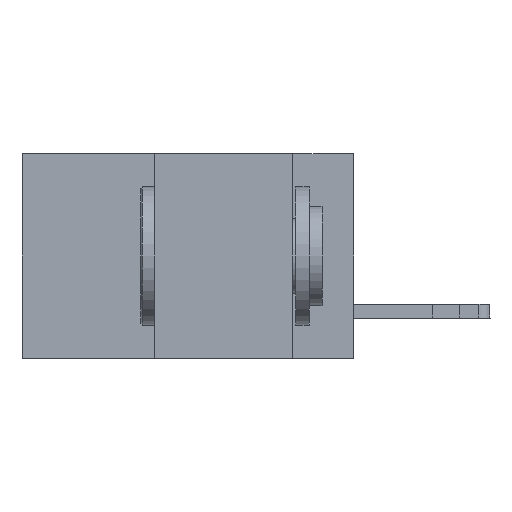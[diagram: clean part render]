
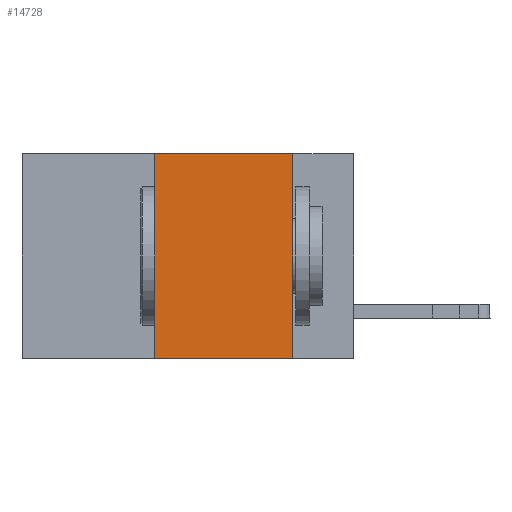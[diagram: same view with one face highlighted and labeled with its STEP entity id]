
A CAD part, left-side view. The second image highlights one B-rep face of the part: STEP entity #14728.
In plain terms, the highlighted planar face has unit normal (-1, 0, 0).
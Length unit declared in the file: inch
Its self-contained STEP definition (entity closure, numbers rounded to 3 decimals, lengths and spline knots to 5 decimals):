
#1623 = DIRECTION ( 'NONE',  ( 1., 0., 0. ) ) ;
#1757 = AXIS2_PLACEMENT_3D ( 'NONE', #15663, #1623, #9814 ) ;
#1800 = VECTOR ( 'NONE', #20126, 39.37008 ) ;
#3189 = LINE ( 'NONE', #13728, #12115 ) ;
#3239 = ORIENTED_EDGE ( 'NONE', *, *, #13617, .F. ) ;
#3322 = LINE ( 'NONE', #13503, #13799 ) ;
#3452 = EDGE_CURVE ( 'NONE', #20125, #24750, #3322, .T. ) ;
#4937 = EDGE_LOOP ( 'NONE', ( #3239, #13744, #5851, #11400 ) ) ;
#5851 = ORIENTED_EDGE ( 'NONE', *, *, #20965, .F. ) ;
#6671 = LINE ( 'NONE', #15623, #1800 ) ;
#7636 = DIRECTION ( 'NONE',  ( 0., -1., 0. ) ) ;
#9814 = DIRECTION ( 'NONE',  ( 0., 0., -1. ) ) ;
#10071 = FACE_OUTER_BOUND ( 'NONE', #4937, .T. ) ;
#11400 = ORIENTED_EDGE ( 'NONE', *, *, #3452, .T. ) ;
#12115 = VECTOR ( 'NONE', #15627, 39.37008 ) ;
#13503 = CARTESIAN_POINT ( 'NONE',  ( 0., 0.6, -0.37 ) ) ;
#13617 = EDGE_CURVE ( 'NONE', #23553, #24750, #6671, .T. ) ;
#13728 = CARTESIAN_POINT ( 'NONE',  ( 0., 0.36, 0. ) ) ;
#13744 = ORIENTED_EDGE ( 'NONE', *, *, #15379, .F. ) ;
#13775 = CARTESIAN_POINT ( 'NONE',  ( 0., 0.36, -0.37 ) ) ;
#13799 = VECTOR ( 'NONE', #7636, 39.37008 ) ;
#14728 = ADVANCED_FACE ( 'NONE', ( #10071 ), #21417, .F. ) ;
#15379 = EDGE_CURVE ( 'NONE', #22194, #23553, #22036, .T. ) ;
#15623 = CARTESIAN_POINT ( 'NONE',  ( 0., 0.11, 0. ) ) ;
#15627 = DIRECTION ( 'NONE',  ( 0., 0., 1. ) ) ;
#15663 = CARTESIAN_POINT ( 'NONE',  ( 0., 0.6, 0. ) ) ;
#16547 = CARTESIAN_POINT ( 'NONE',  ( 0., 0.11, -0.37 ) ) ;
#19890 = CARTESIAN_POINT ( 'NONE',  ( 0., 0.36, 0. ) ) ;
#20125 = VERTEX_POINT ( 'NONE', #13775 ) ;
#20126 = DIRECTION ( 'NONE',  ( 0., 0., -1. ) ) ;
#20227 = DIRECTION ( 'NONE',  ( 0., -1., 0. ) ) ;
#20965 = EDGE_CURVE ( 'NONE', #20125, #22194, #3189, .T. ) ;
#21417 = PLANE ( 'NONE',  #1757 ) ;
#22036 = LINE ( 'NONE', #24097, #23843 ) ;
#22194 = VERTEX_POINT ( 'NONE', #19890 ) ;
#23553 = VERTEX_POINT ( 'NONE', #25076 ) ;
#23843 = VECTOR ( 'NONE', #20227, 39.37008 ) ;
#24097 = CARTESIAN_POINT ( 'NONE',  ( 0., 0.6, 0. ) ) ;
#24750 = VERTEX_POINT ( 'NONE', #16547 ) ;
#25076 = CARTESIAN_POINT ( 'NONE',  ( 0., 0.11, 0. ) ) ;
